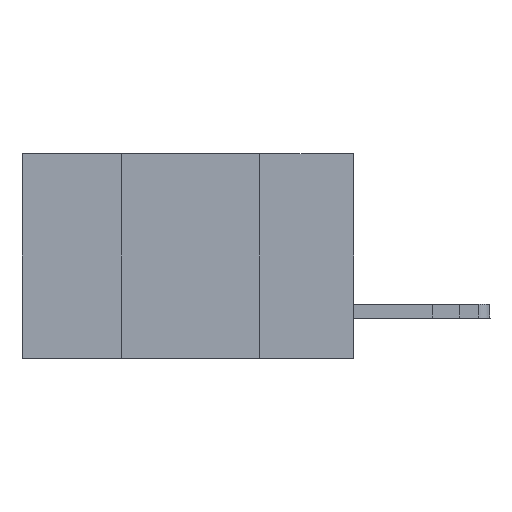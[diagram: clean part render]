
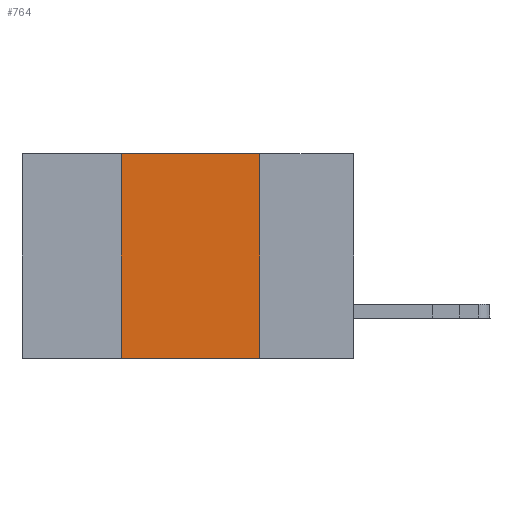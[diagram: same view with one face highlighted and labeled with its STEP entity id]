
A CAD part, left-side view. The second image highlights one B-rep face of the part: STEP entity #764.
In plain terms, the highlighted planar face has unit normal (-1, 0, 0).
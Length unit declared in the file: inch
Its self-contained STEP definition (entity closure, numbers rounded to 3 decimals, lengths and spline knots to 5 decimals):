
#428 = VECTOR ( 'NONE', #1888, 39.37008 ) ;
#609 = EDGE_CURVE ( 'NONE', #20066, #18104, #804, .T. ) ;
#764 = ADVANCED_FACE ( 'NONE', ( #2970 ), #1930, .F. ) ;
#804 = LINE ( 'NONE', #13164, #22127 ) ;
#906 = CARTESIAN_POINT ( 'NONE',  ( 0., 0.42, 0. ) ) ;
#1888 = DIRECTION ( 'NONE',  ( 0., -1., 0. ) ) ;
#1930 = PLANE ( 'NONE',  #18359 ) ;
#2740 = VERTEX_POINT ( 'NONE', #10492 ) ;
#2970 = FACE_OUTER_BOUND ( 'NONE', #14498, .T. ) ;
#3339 = ORIENTED_EDGE ( 'NONE', *, *, #14247, .F. ) ;
#3528 = ORIENTED_EDGE ( 'NONE', *, *, #16113, .T. ) ;
#5468 = DIRECTION ( 'NONE',  ( 0., -1., 0. ) ) ;
#6512 = CARTESIAN_POINT ( 'NONE',  ( 0., 0.42, -0.37 ) ) ;
#6744 = ORIENTED_EDGE ( 'NONE', *, *, #609, .F. ) ;
#8850 = LINE ( 'NONE', #16976, #21522 ) ;
#10492 = CARTESIAN_POINT ( 'NONE',  ( 0., 0.17, 0. ) ) ;
#10579 = DIRECTION ( 'NONE',  ( 1., 0., 0. ) ) ;
#12378 = CARTESIAN_POINT ( 'NONE',  ( 0., 0.6, 0. ) ) ;
#13164 = CARTESIAN_POINT ( 'NONE',  ( 0., 0.42, 0. ) ) ;
#13991 = ORIENTED_EDGE ( 'NONE', *, *, #21840, .F. ) ;
#14111 = DIRECTION ( 'NONE',  ( 0., 0., -1. ) ) ;
#14247 = EDGE_CURVE ( 'NONE', #18104, #2740, #16125, .T. ) ;
#14498 = EDGE_LOOP ( 'NONE', ( #13991, #3339, #6744, #3528 ) ) ;
#14632 = CARTESIAN_POINT ( 'NONE',  ( 0., 0.17, -0.37 ) ) ;
#15471 = CARTESIAN_POINT ( 'NONE',  ( 0., 0.6, 0. ) ) ;
#15518 = DIRECTION ( 'NONE',  ( 0., 0., -1. ) ) ;
#16113 = EDGE_CURVE ( 'NONE', #20066, #18397, #18792, .T. ) ;
#16125 = LINE ( 'NONE', #15471, #16668 ) ;
#16668 = VECTOR ( 'NONE', #5468, 39.37008 ) ;
#16976 = CARTESIAN_POINT ( 'NONE',  ( 0., 0.17, 0. ) ) ;
#17210 = CARTESIAN_POINT ( 'NONE',  ( 0., 0.6, -0.37 ) ) ;
#18104 = VERTEX_POINT ( 'NONE', #906 ) ;
#18359 = AXIS2_PLACEMENT_3D ( 'NONE', #12378, #10579, #14111 ) ;
#18397 = VERTEX_POINT ( 'NONE', #14632 ) ;
#18792 = LINE ( 'NONE', #17210, #428 ) ;
#20066 = VERTEX_POINT ( 'NONE', #6512 ) ;
#21522 = VECTOR ( 'NONE', #15518, 39.37008 ) ;
#21840 = EDGE_CURVE ( 'NONE', #2740, #18397, #8850, .T. ) ;
#21891 = DIRECTION ( 'NONE',  ( 0., 0., 1. ) ) ;
#22127 = VECTOR ( 'NONE', #21891, 39.37008 ) ;
